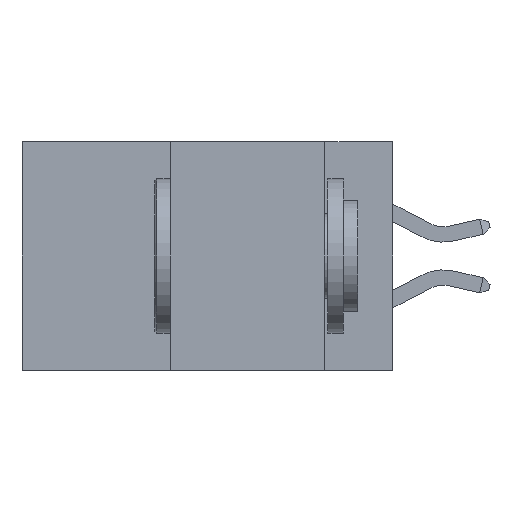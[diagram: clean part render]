
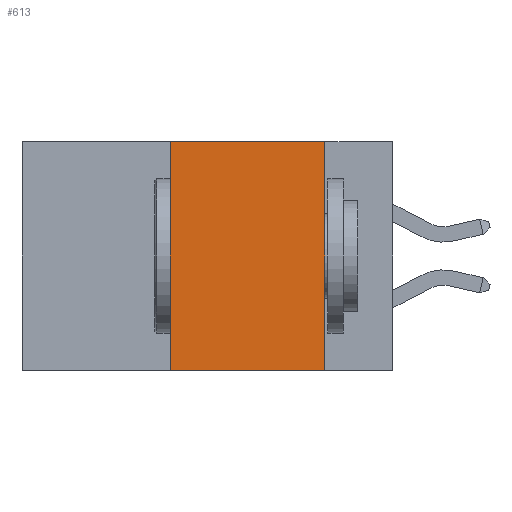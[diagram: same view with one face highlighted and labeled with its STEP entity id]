
A CAD part, left-side view. The second image highlights one B-rep face of the part: STEP entity #613.
In plain terms, the highlighted planar face has unit normal (-1, 0, 0).
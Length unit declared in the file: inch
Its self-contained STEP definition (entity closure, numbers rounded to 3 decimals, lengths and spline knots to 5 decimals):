
#9 = ORIENTED_EDGE ( 'NONE', *, *, #2063, .T. ) ;
#413 = DIRECTION ( 'NONE',  ( 0., -1., 0. ) ) ;
#459 = DIRECTION ( 'NONE',  ( 0., 0., -1. ) ) ;
#599 = EDGE_CURVE ( 'NONE', #5540, #6077, #8228, .T. ) ;
#613 = ADVANCED_FACE ( 'NONE', ( #5830 ), #3626, .F. ) ;
#698 = VECTOR ( 'NONE', #4831, 39.37008 ) ;
#708 = VECTOR ( 'NONE', #5496, 39.37008 ) ;
#1846 = VECTOR ( 'NONE', #7849, 39.37008 ) ;
#1997 = VERTEX_POINT ( 'NONE', #2941 ) ;
#2063 = EDGE_CURVE ( 'NONE', #1997, #8055, #5026, .T. ) ;
#2643 = ORIENTED_EDGE ( 'NONE', *, *, #2659, .F. ) ;
#2659 = EDGE_CURVE ( 'NONE', #1997, #5540, #9999, .T. ) ;
#2941 = CARTESIAN_POINT ( 'NONE',  ( 0., 0.36, -0.37 ) ) ;
#3105 = CARTESIAN_POINT ( 'NONE',  ( 0., 0.11, 0. ) ) ;
#3626 = PLANE ( 'NONE',  #5241 ) ;
#3859 = LINE ( 'NONE', #5343, #708 ) ;
#4388 = VECTOR ( 'NONE', #413, 39.37008 ) ;
#4547 = DIRECTION ( 'NONE',  ( 1., 0., 0. ) ) ;
#4777 = ORIENTED_EDGE ( 'NONE', *, *, #5871, .F. ) ;
#4831 = DIRECTION ( 'NONE',  ( 0., 0., 1. ) ) ;
#5026 = LINE ( 'NONE', #9339, #4388 ) ;
#5241 = AXIS2_PLACEMENT_3D ( 'NONE', #9411, #4547, #459 ) ;
#5343 = CARTESIAN_POINT ( 'NONE',  ( 0., 0.11, 0. ) ) ;
#5496 = DIRECTION ( 'NONE',  ( 0., 0., -1. ) ) ;
#5540 = VERTEX_POINT ( 'NONE', #6710 ) ;
#5830 = FACE_OUTER_BOUND ( 'NONE', #6172, .T. ) ;
#5871 = EDGE_CURVE ( 'NONE', #6077, #8055, #3859, .T. ) ;
#5935 = ORIENTED_EDGE ( 'NONE', *, *, #599, .F. ) ;
#6077 = VERTEX_POINT ( 'NONE', #3105 ) ;
#6172 = EDGE_LOOP ( 'NONE', ( #4777, #5935, #2643, #9 ) ) ;
#6710 = CARTESIAN_POINT ( 'NONE',  ( 0., 0.36, 0. ) ) ;
#7849 = DIRECTION ( 'NONE',  ( 0., -1., 0. ) ) ;
#8055 = VERTEX_POINT ( 'NONE', #10318 ) ;
#8228 = LINE ( 'NONE', #8534, #1846 ) ;
#8534 = CARTESIAN_POINT ( 'NONE',  ( 0., 0.6, 0. ) ) ;
#9339 = CARTESIAN_POINT ( 'NONE',  ( 0., 0.6, -0.37 ) ) ;
#9411 = CARTESIAN_POINT ( 'NONE',  ( 0., 0.6, 0. ) ) ;
#9735 = CARTESIAN_POINT ( 'NONE',  ( 0., 0.36, 0. ) ) ;
#9999 = LINE ( 'NONE', #9735, #698 ) ;
#10318 = CARTESIAN_POINT ( 'NONE',  ( 0., 0.11, -0.37 ) ) ;
